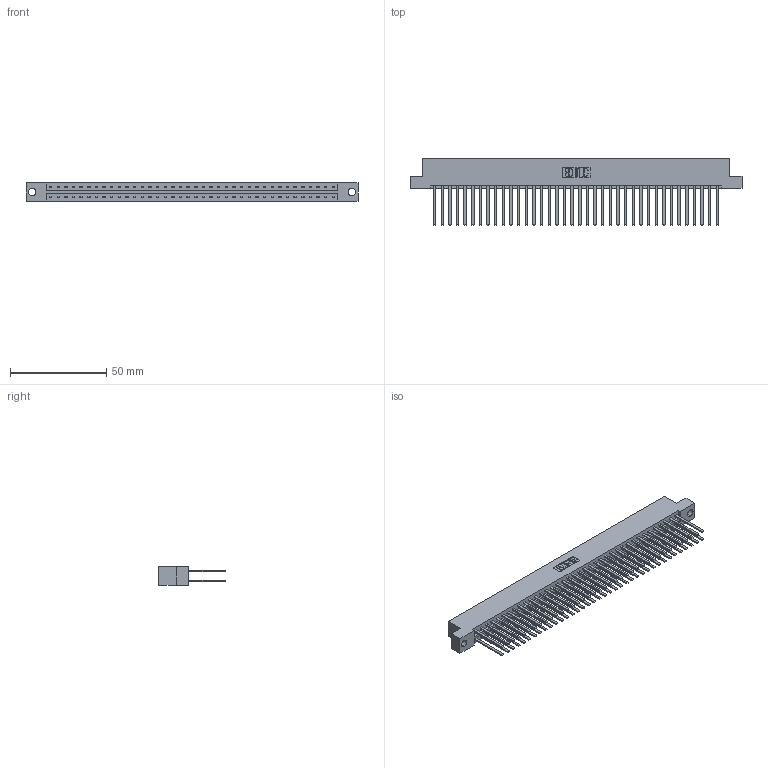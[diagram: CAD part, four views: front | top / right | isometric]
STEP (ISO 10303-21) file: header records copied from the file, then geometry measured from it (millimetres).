
FILE_DESCRIPTION (( 'STEP AP203' ), '1' );
FILE_NAME ('833-076-544-204.STEP', '2020-06-05T18:39:22', ( '' ), ( '' ), 'SwSTEP 2.0', 'SolidWorks 2020', '' );
FILE_SCHEMA (( 'CONFIG_CONTROL_DESIGN' ));
Length unit declared in the file: inch
Products named in the file (3): 833-076-544-204; 345-292-001_345-293-144; 833 Part_Flush - .156 Dia - TH
Assembly tree (77 placements, depth 2):
  833-076-544-204
    833 Part_Flush - .156 Dia - TH
    345-292-001_345-293-144  x76
Bounding box: 172.11 x 34.3 x 9.4 mm (x, y, z)
Volume: 18511.6 mm3; surface area: 25072 mm2
Topology: 77 solids, 77 shells, 3610 faces, 10723 edges, 7046 vertices
Faces by surface type: plane 2502, cylinder 1108
Entity records: 24783 total; most frequent: CARTESIAN_POINT 4110, ORIENTED_EDGE 4046, DIRECTION 3515, EDGE_CURVE 2023, LINE 1899, VECTOR 1899, VERTEX_POINT 1346, AXIS2_PLACEMENT_3D 808
